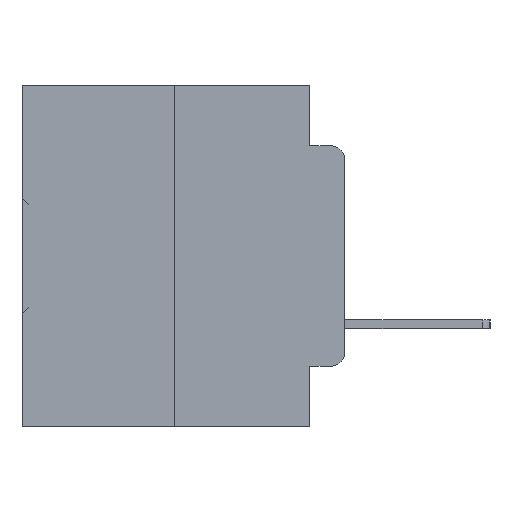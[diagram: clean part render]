
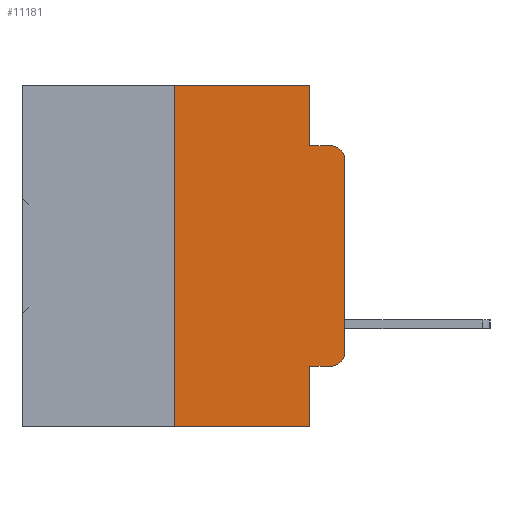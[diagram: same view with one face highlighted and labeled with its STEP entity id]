
A CAD part, left-side view. The second image highlights one B-rep face of the part: STEP entity #11181.
In plain terms, the highlighted planar face has unit normal (-1, 0, 0).
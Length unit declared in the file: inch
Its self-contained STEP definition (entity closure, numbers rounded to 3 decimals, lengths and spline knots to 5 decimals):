
#204 = EDGE_CURVE ( 'NONE', #24164, #30348, #5039, .T. ) ;
#330 = CARTESIAN_POINT ( 'NONE',  ( 0., 0.473, 0. ) ) ;
#921 = CARTESIAN_POINT ( 'NONE',  ( 0., 0.051, -0.0885 ) ) ;
#1676 = EDGE_CURVE ( 'NONE', #30348, #17473, #22003, .T. ) ;
#2185 = VERTEX_POINT ( 'NONE', #24273 ) ;
#2868 = DIRECTION ( 'NONE',  ( 0., -1., 0. ) ) ;
#3614 = DIRECTION ( 'NONE',  ( 0., 0., -1. ) ) ;
#3989 = AXIS2_PLACEMENT_3D ( 'NONE', #330, #22579, #5911 ) ;
#4063 = ORIENTED_EDGE ( 'NONE', *, *, #33560, .F. ) ;
#5039 = CIRCLE ( 'NONE', #34885, 0.02 ) ;
#5823 = ORIENTED_EDGE ( 'NONE', *, *, #16550, .F. ) ;
#5911 = DIRECTION ( 'NONE',  ( 0., 0., -1. ) ) ;
#6211 = DIRECTION ( 'NONE',  ( 0., 0., -1. ) ) ;
#6215 = DIRECTION ( 'NONE',  ( 0., 0., 1. ) ) ;
#6677 = LINE ( 'NONE', #11978, #35026 ) ;
#6742 = DIRECTION ( 'NONE',  ( 0., 0., 1. ) ) ;
#6800 = VECTOR ( 'NONE', #6211, 39.37008 ) ;
#7141 = ORIENTED_EDGE ( 'NONE', *, *, #28573, .F. ) ;
#7359 = DIRECTION ( 'NONE',  ( 0., 0., -1. ) ) ;
#7441 = DIRECTION ( 'NONE',  ( -1., 0., 0. ) ) ;
#7483 = CARTESIAN_POINT ( 'NONE',  ( 0., 0.02, -0.3915 ) ) ;
#7605 = ORIENTED_EDGE ( 'NONE', *, *, #12982, .F. ) ;
#7623 = CARTESIAN_POINT ( 'NONE',  ( 0., 0.051, -0.4115 ) ) ;
#9470 = EDGE_CURVE ( 'NONE', #17473, #20002, #10529, .T. ) ;
#9796 = ORIENTED_EDGE ( 'NONE', *, *, #18610, .F. ) ;
#9976 = CARTESIAN_POINT ( 'NONE',  ( 0., 0., -0.1085 ) ) ;
#10435 = DIRECTION ( 'NONE',  ( 0., -1., 0. ) ) ;
#10529 = CIRCLE ( 'NONE', #27438, 0.02 ) ;
#11181 = ADVANCED_FACE ( 'NONE', ( #12141 ), #17035, .F. ) ;
#11299 = DIRECTION ( 'NONE',  ( 0., -1., 0. ) ) ;
#11978 = CARTESIAN_POINT ( 'NONE',  ( 0., 0.051, 0. ) ) ;
#12141 = FACE_OUTER_BOUND ( 'NONE', #30174, .T. ) ;
#12982 = EDGE_CURVE ( 'NONE', #26102, #26241, #35138, .T. ) ;
#13111 = CARTESIAN_POINT ( 'NONE',  ( 0., 0.02, -0.0885 ) ) ;
#13935 = DIRECTION ( 'NONE',  ( 0., -1., 0. ) ) ;
#14389 = CARTESIAN_POINT ( 'NONE',  ( 0., 0.051, -0.5 ) ) ;
#14478 = DIRECTION ( 'NONE',  ( -1., 0., 0. ) ) ;
#14555 = VERTEX_POINT ( 'NONE', #921 ) ;
#15648 = EDGE_CURVE ( 'NONE', #32460, #26241, #16903, .T. ) ;
#15954 = VECTOR ( 'NONE', #6742, 39.37008 ) ;
#16550 = EDGE_CURVE ( 'NONE', #32460, #34503, #16831, .T. ) ;
#16640 = EDGE_CURVE ( 'NONE', #26102, #24164, #27151, .T. ) ;
#16769 = ORIENTED_EDGE ( 'NONE', *, *, #16640, .T. ) ;
#16831 = LINE ( 'NONE', #23413, #15954 ) ;
#16903 = LINE ( 'NONE', #22369, #23398 ) ;
#17035 = PLANE ( 'NONE',  #3989 ) ;
#17473 = VERTEX_POINT ( 'NONE', #9976 ) ;
#17533 = CARTESIAN_POINT ( 'NONE',  ( 0., 0., 0. ) ) ;
#18498 = ORIENTED_EDGE ( 'NONE', *, *, #204, .T. ) ;
#18610 = EDGE_CURVE ( 'NONE', #2185, #14555, #6677, .T. ) ;
#20002 = VERTEX_POINT ( 'NONE', #13111 ) ;
#20105 = CARTESIAN_POINT ( 'NONE',  ( 0., 0.051, 0. ) ) ;
#20214 = ORIENTED_EDGE ( 'NONE', *, *, #9470, .T. ) ;
#22003 = LINE ( 'NONE', #17533, #35548 ) ;
#22108 = CARTESIAN_POINT ( 'NONE',  ( 0., 0.051, -0.4115 ) ) ;
#22369 = CARTESIAN_POINT ( 'NONE',  ( 0., 0.473, -0.5 ) ) ;
#22579 = DIRECTION ( 'NONE',  ( 1., 0., 0. ) ) ;
#23398 = VECTOR ( 'NONE', #2868, 39.37008 ) ;
#23413 = CARTESIAN_POINT ( 'NONE',  ( 0., 0.25, 0. ) ) ;
#24055 = CARTESIAN_POINT ( 'NONE',  ( 0., 0.25, 0. ) ) ;
#24164 = VERTEX_POINT ( 'NONE', #24430 ) ;
#24273 = CARTESIAN_POINT ( 'NONE',  ( 0., 0.051, 0. ) ) ;
#24430 = CARTESIAN_POINT ( 'NONE',  ( 0., 0.02, -0.4115 ) ) ;
#25481 = CARTESIAN_POINT ( 'NONE',  ( 0., 0.25, -0.5 ) ) ;
#25798 = ORIENTED_EDGE ( 'NONE', *, *, #1676, .T. ) ;
#26025 = VECTOR ( 'NONE', #13935, 39.37008 ) ;
#26102 = VERTEX_POINT ( 'NONE', #22108 ) ;
#26241 = VERTEX_POINT ( 'NONE', #14389 ) ;
#27151 = LINE ( 'NONE', #7623, #34293 ) ;
#27438 = AXIS2_PLACEMENT_3D ( 'NONE', #30901, #14478, #33585 ) ;
#28497 = CARTESIAN_POINT ( 'NONE',  ( 0., 0., -0.3915 ) ) ;
#28573 = EDGE_CURVE ( 'NONE', #14555, #20002, #33079, .T. ) ;
#28778 = ORIENTED_EDGE ( 'NONE', *, *, #15648, .T. ) ;
#30174 = EDGE_LOOP ( 'NONE', ( #25798, #20214, #7141, #9796, #4063, #5823, #28778, #7605, #16769, #18498 ) ) ;
#30348 = VERTEX_POINT ( 'NONE', #28497 ) ;
#30536 = CARTESIAN_POINT ( 'NONE',  ( 0., 0.051, -0.0885 ) ) ;
#30901 = CARTESIAN_POINT ( 'NONE',  ( 0., 0.02, -0.1085 ) ) ;
#32242 = VECTOR ( 'NONE', #11299, 39.37008 ) ;
#32460 = VERTEX_POINT ( 'NONE', #25481 ) ;
#33065 = CARTESIAN_POINT ( 'NONE',  ( 0., 0.473, 0. ) ) ;
#33079 = LINE ( 'NONE', #30536, #32242 ) ;
#33178 = LINE ( 'NONE', #33065, #26025 ) ;
#33560 = EDGE_CURVE ( 'NONE', #34503, #2185, #33178, .T. ) ;
#33585 = DIRECTION ( 'NONE',  ( 0., 0., -1. ) ) ;
#34293 = VECTOR ( 'NONE', #10435, 39.37008 ) ;
#34503 = VERTEX_POINT ( 'NONE', #24055 ) ;
#34885 = AXIS2_PLACEMENT_3D ( 'NONE', #7483, #7441, #7359 ) ;
#35026 = VECTOR ( 'NONE', #3614, 39.37008 ) ;
#35138 = LINE ( 'NONE', #20105, #6800 ) ;
#35548 = VECTOR ( 'NONE', #6215, 39.37008 ) ;
